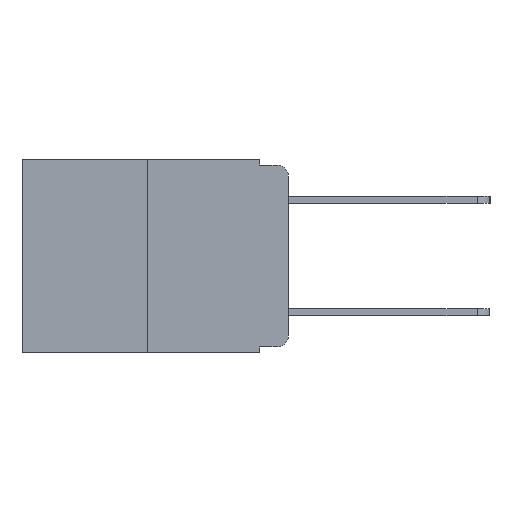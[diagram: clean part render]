
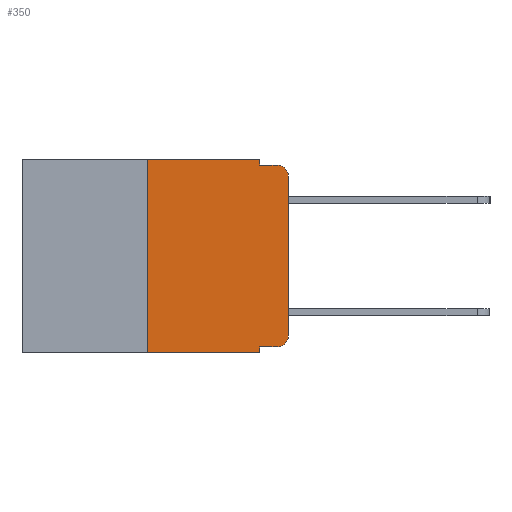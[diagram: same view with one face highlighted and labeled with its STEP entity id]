
A CAD part, left-side view. The second image highlights one B-rep face of the part: STEP entity #350.
In plain terms, the highlighted planar face has unit normal (-1, 0, 0).
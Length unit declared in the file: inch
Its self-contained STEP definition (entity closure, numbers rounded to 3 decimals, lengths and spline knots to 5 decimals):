
#87 = ORIENTED_EDGE ( 'NONE', *, *, #7902, .F. ) ;
#93 = LINE ( 'NONE', #958, #2827 ) ;
#350 = ADVANCED_FACE ( 'NONE', ( #710 ), #7799, .F. ) ;
#448 = ORIENTED_EDGE ( 'NONE', *, *, #6713, .F. ) ;
#710 = FACE_OUTER_BOUND ( 'NONE', #10190, .T. ) ;
#958 = CARTESIAN_POINT ( 'NONE',  ( 0., 0.25, 0. ) ) ;
#1121 = VECTOR ( 'NONE', #2727, 39.37008 ) ;
#1373 = LINE ( 'NONE', #8494, #12732 ) ;
#1510 = AXIS2_PLACEMENT_3D ( 'NONE', #3436, #9511, #3959 ) ;
#1703 = VERTEX_POINT ( 'NONE', #6707 ) ;
#1800 = CARTESIAN_POINT ( 'NONE',  ( 0., 0.02, -0.313 ) ) ;
#2022 = AXIS2_PLACEMENT_3D ( 'NONE', #5324, #12385, #6441 ) ;
#2243 = LINE ( 'NONE', #4432, #12845 ) ;
#2297 = ORIENTED_EDGE ( 'NONE', *, *, #12551, .T. ) ;
#2727 = DIRECTION ( 'NONE',  ( 0., -1., 0. ) ) ;
#2827 = VECTOR ( 'NONE', #4332, 39.37008 ) ;
#2929 = DIRECTION ( 'NONE',  ( 0., 0., -1. ) ) ;
#3065 = VECTOR ( 'NONE', #11397, 39.37008 ) ;
#3152 = VECTOR ( 'NONE', #5823, 39.37008 ) ;
#3166 = ORIENTED_EDGE ( 'NONE', *, *, #9251, .F. ) ;
#3375 = DIRECTION ( 'NONE',  ( 0., 0., -1. ) ) ;
#3436 = CARTESIAN_POINT ( 'NONE',  ( 0., 0.473, 0. ) ) ;
#3635 = VERTEX_POINT ( 'NONE', #11494 ) ;
#3923 = CARTESIAN_POINT ( 'NONE',  ( 0., 0.051, -0.343 ) ) ;
#3959 = DIRECTION ( 'NONE',  ( 0., 0., -1. ) ) ;
#4094 = LINE ( 'NONE', #12909, #1121 ) ;
#4201 = CARTESIAN_POINT ( 'NONE',  ( 0., 0.051, -0.333 ) ) ;
#4218 = CARTESIAN_POINT ( 'NONE',  ( 0., 0., -0.313 ) ) ;
#4332 = DIRECTION ( 'NONE',  ( 0., 0., 1. ) ) ;
#4432 = CARTESIAN_POINT ( 'NONE',  ( 0., 0.473, 0. ) ) ;
#4959 = VERTEX_POINT ( 'NONE', #6633 ) ;
#5112 = EDGE_CURVE ( 'NONE', #8245, #8404, #11349, .T. ) ;
#5324 = CARTESIAN_POINT ( 'NONE',  ( 0., 0.02, -0.03 ) ) ;
#5333 = ORIENTED_EDGE ( 'NONE', *, *, #5112, .T. ) ;
#5415 = DIRECTION ( 'NONE',  ( 0., 0., -1. ) ) ;
#5645 = VECTOR ( 'NONE', #11356, 39.37008 ) ;
#5794 = AXIS2_PLACEMENT_3D ( 'NONE', #1800, #9180, #2929 ) ;
#5823 = DIRECTION ( 'NONE',  ( 0., 0., 1. ) ) ;
#5931 = LINE ( 'NONE', #8409, #3065 ) ;
#6234 = LINE ( 'NONE', #9595, #7982 ) ;
#6441 = DIRECTION ( 'NONE',  ( 0., 0., -1. ) ) ;
#6461 = VERTEX_POINT ( 'NONE', #8282 ) ;
#6567 = EDGE_CURVE ( 'NONE', #8404, #10301, #11794, .T. ) ;
#6633 = CARTESIAN_POINT ( 'NONE',  ( 0., 0.25, 0. ) ) ;
#6707 = CARTESIAN_POINT ( 'NONE',  ( 0., 0.25, -0.343 ) ) ;
#6713 = EDGE_CURVE ( 'NONE', #4959, #10338, #2243, .T. ) ;
#6891 = CARTESIAN_POINT ( 'NONE',  ( 0., 0., 0. ) ) ;
#7001 = ORIENTED_EDGE ( 'NONE', *, *, #10579, .F. ) ;
#7122 = CARTESIAN_POINT ( 'NONE',  ( 0., 0.02, -0.01 ) ) ;
#7129 = VERTEX_POINT ( 'NONE', #3923 ) ;
#7307 = ORIENTED_EDGE ( 'NONE', *, *, #9101, .T. ) ;
#7799 = PLANE ( 'NONE',  #1510 ) ;
#7902 = EDGE_CURVE ( 'NONE', #6461, #10301, #4094, .T. ) ;
#7943 = ORIENTED_EDGE ( 'NONE', *, *, #13203, .T. ) ;
#7982 = VECTOR ( 'NONE', #3375, 39.37008 ) ;
#8052 = LINE ( 'NONE', #4201, #5645 ) ;
#8245 = VERTEX_POINT ( 'NONE', #4218 ) ;
#8282 = CARTESIAN_POINT ( 'NONE',  ( 0., 0.051, -0.01 ) ) ;
#8404 = VERTEX_POINT ( 'NONE', #10590 ) ;
#8409 = CARTESIAN_POINT ( 'NONE',  ( 0., 0.473, -0.343 ) ) ;
#8420 = ORIENTED_EDGE ( 'NONE', *, *, #6567, .T. ) ;
#8494 = CARTESIAN_POINT ( 'NONE',  ( 0., 0.051, 0. ) ) ;
#9101 = EDGE_CURVE ( 'NONE', #1703, #7129, #5931, .T. ) ;
#9180 = DIRECTION ( 'NONE',  ( -1., 0., 0. ) ) ;
#9251 = EDGE_CURVE ( 'NONE', #10338, #6461, #6234, .T. ) ;
#9511 = DIRECTION ( 'NONE',  ( 1., 0., 0. ) ) ;
#9537 = CARTESIAN_POINT ( 'NONE',  ( 0., 0.02, -0.333 ) ) ;
#9595 = CARTESIAN_POINT ( 'NONE',  ( 0., 0.051, 0. ) ) ;
#9988 = ORIENTED_EDGE ( 'NONE', *, *, #11240, .F. ) ;
#10190 = EDGE_LOOP ( 'NONE', ( #5333, #8420, #87, #3166, #448, #7001, #7307, #9988, #2297, #7943 ) ) ;
#10210 = CARTESIAN_POINT ( 'NONE',  ( 0., 0.051, 0. ) ) ;
#10301 = VERTEX_POINT ( 'NONE', #7122 ) ;
#10338 = VERTEX_POINT ( 'NONE', #10210 ) ;
#10579 = EDGE_CURVE ( 'NONE', #1703, #4959, #93, .T. ) ;
#10590 = CARTESIAN_POINT ( 'NONE',  ( 0., 0., -0.03 ) ) ;
#11240 = EDGE_CURVE ( 'NONE', #3635, #7129, #1373, .T. ) ;
#11349 = LINE ( 'NONE', #6891, #3152 ) ;
#11356 = DIRECTION ( 'NONE',  ( 0., -1., 0. ) ) ;
#11397 = DIRECTION ( 'NONE',  ( 0., -1., 0. ) ) ;
#11494 = CARTESIAN_POINT ( 'NONE',  ( 0., 0.051, -0.333 ) ) ;
#11794 = CIRCLE ( 'NONE', #2022, 0.02 ) ;
#12385 = DIRECTION ( 'NONE',  ( -1., 0., 0. ) ) ;
#12551 = EDGE_CURVE ( 'NONE', #3635, #13398, #8052, .T. ) ;
#12732 = VECTOR ( 'NONE', #5415, 39.37008 ) ;
#12835 = CIRCLE ( 'NONE', #5794, 0.02 ) ;
#12845 = VECTOR ( 'NONE', #13552, 39.37008 ) ;
#12909 = CARTESIAN_POINT ( 'NONE',  ( 0., 0.051, -0.01 ) ) ;
#13203 = EDGE_CURVE ( 'NONE', #13398, #8245, #12835, .T. ) ;
#13398 = VERTEX_POINT ( 'NONE', #9537 ) ;
#13552 = DIRECTION ( 'NONE',  ( 0., -1., 0. ) ) ;
